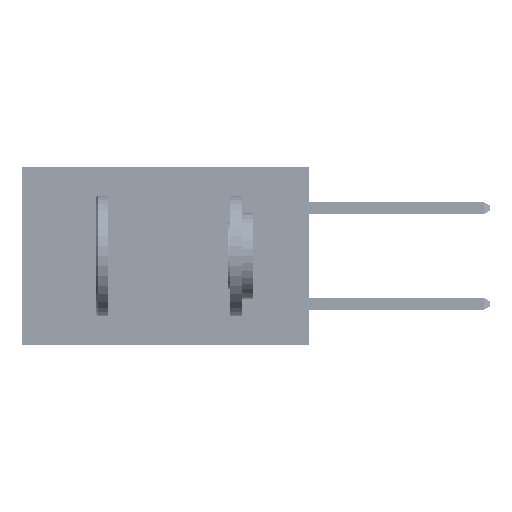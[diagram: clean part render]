
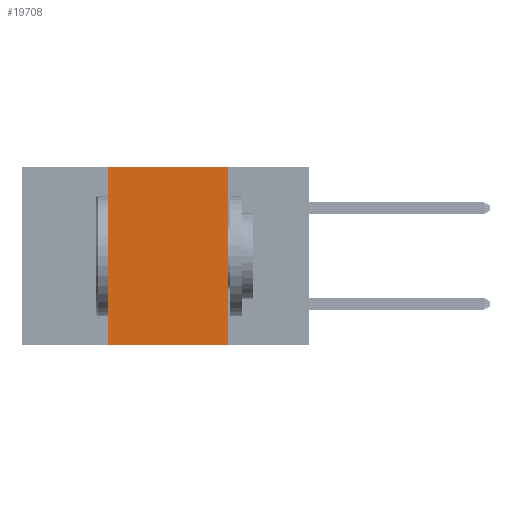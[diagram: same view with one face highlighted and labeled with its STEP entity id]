
A CAD part, left-side view. The second image highlights one B-rep face of the part: STEP entity #19708.
In plain terms, the highlighted planar face has unit normal (-1, 0, 0).
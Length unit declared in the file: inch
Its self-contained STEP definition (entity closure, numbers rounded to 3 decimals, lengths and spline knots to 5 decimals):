
#1368 = VERTEX_POINT ( 'NONE', #22838 ) ;
#2147 = PLANE ( 'NONE',  #46809 ) ;
#3863 = EDGE_CURVE ( 'NONE', #1368, #41640, #21613, .T. ) ;
#4621 = CARTESIAN_POINT ( 'NONE',  ( 0., 0.6, -0.37 ) ) ;
#6420 = DIRECTION ( 'NONE',  ( 1., 0., 0. ) ) ;
#7497 = LINE ( 'NONE', #46440, #17331 ) ;
#8721 = ORIENTED_EDGE ( 'NONE', *, *, #10635, .T. ) ;
#10635 = EDGE_CURVE ( 'NONE', #41938, #28550, #37148, .T. ) ;
#10772 = FACE_OUTER_BOUND ( 'NONE', #45182, .T. ) ;
#12971 = CARTESIAN_POINT ( 'NONE',  ( 0., 0.17, -0.37 ) ) ;
#14756 = DIRECTION ( 'NONE',  ( 0., -1., 0. ) ) ;
#17331 = VECTOR ( 'NONE', #18018, 39.37008 ) ;
#18018 = DIRECTION ( 'NONE',  ( 0., 0., -1. ) ) ;
#19554 = EDGE_CURVE ( 'NONE', #41640, #28550, #7497, .T. ) ;
#19708 = ADVANCED_FACE ( 'NONE', ( #10772 ), #2147, .F. ) ;
#20451 = ORIENTED_EDGE ( 'NONE', *, *, #24607, .F. ) ;
#21613 = LINE ( 'NONE', #43296, #32481 ) ;
#21825 = DIRECTION ( 'NONE',  ( 0., 0., 1. ) ) ;
#22838 = CARTESIAN_POINT ( 'NONE',  ( 0., 0.42, 0. ) ) ;
#24607 = EDGE_CURVE ( 'NONE', #41938, #1368, #33812, .T. ) ;
#25609 = DIRECTION ( 'NONE',  ( 0., -1., 0. ) ) ;
#25955 = CARTESIAN_POINT ( 'NONE',  ( 0., 0.42, 0. ) ) ;
#28550 = VERTEX_POINT ( 'NONE', #12971 ) ;
#30282 = CARTESIAN_POINT ( 'NONE',  ( 0., 0.42, -0.37 ) ) ;
#31208 = CARTESIAN_POINT ( 'NONE',  ( 0., 0.6, 0. ) ) ;
#31917 = ORIENTED_EDGE ( 'NONE', *, *, #19554, .F. ) ;
#32481 = VECTOR ( 'NONE', #14756, 39.37008 ) ;
#33197 = ORIENTED_EDGE ( 'NONE', *, *, #3863, .F. ) ;
#33812 = LINE ( 'NONE', #25955, #45840 ) ;
#35314 = DIRECTION ( 'NONE',  ( 0., 0., -1. ) ) ;
#37148 = LINE ( 'NONE', #4621, #46647 ) ;
#41640 = VERTEX_POINT ( 'NONE', #47923 ) ;
#41938 = VERTEX_POINT ( 'NONE', #30282 ) ;
#43296 = CARTESIAN_POINT ( 'NONE',  ( 0., 0.6, 0. ) ) ;
#45182 = EDGE_LOOP ( 'NONE', ( #31917, #33197, #20451, #8721 ) ) ;
#45840 = VECTOR ( 'NONE', #21825, 39.37008 ) ;
#46440 = CARTESIAN_POINT ( 'NONE',  ( 0., 0.17, 0. ) ) ;
#46647 = VECTOR ( 'NONE', #25609, 39.37008 ) ;
#46809 = AXIS2_PLACEMENT_3D ( 'NONE', #31208, #6420, #35314 ) ;
#47923 = CARTESIAN_POINT ( 'NONE',  ( 0., 0.17, 0. ) ) ;
